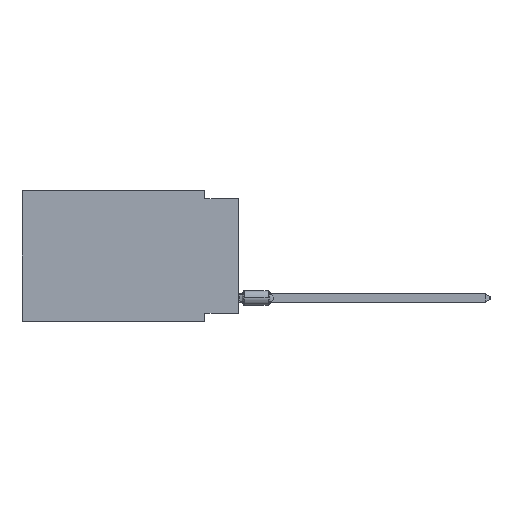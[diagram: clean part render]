
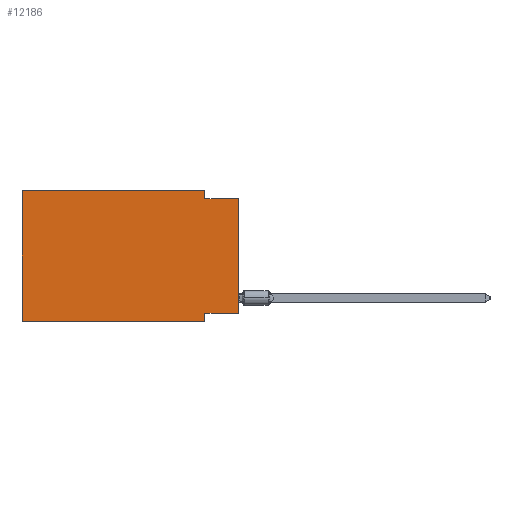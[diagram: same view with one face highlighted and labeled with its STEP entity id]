
A CAD part, left-side view. The second image highlights one B-rep face of the part: STEP entity #12186.
In plain terms, the highlighted planar face has unit normal (-1, 0, 0).
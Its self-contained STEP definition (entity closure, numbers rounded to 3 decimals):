
#16 = CARTESIAN_POINT ( 'NONE',  ( 0., 0., -0.635 ) ) ;
#1553 = DIRECTION ( 'NONE',  ( 0., 0., 1. ) ) ;
#1969 = EDGE_LOOP ( 'NONE', ( #14533, #6865, #28409, #47356, #5239, #27205, #57407, #11912 ) ) ;
#5239 = ORIENTED_EDGE ( 'NONE', *, *, #33198, .F. ) ;
#5409 = DIRECTION ( 'NONE',  ( 0., -1., 0. ) ) ;
#6129 = CARTESIAN_POINT ( 'NONE',  ( 0., 0., 0. ) ) ;
#6865 = ORIENTED_EDGE ( 'NONE', *, *, #43798, .F. ) ;
#7364 = VECTOR ( 'NONE', #43977, 1000. ) ;
#9691 = CARTESIAN_POINT ( 'NONE',  ( 0., 2.54, 0. ) ) ;
#11912 = ORIENTED_EDGE ( 'NONE', *, *, #61430, .F. ) ;
#12186 = ADVANCED_FACE ( 'NONE', ( #35207 ), #50902, .F. ) ;
#12616 = VECTOR ( 'NONE', #14151, 1000. ) ;
#13844 = DIRECTION ( 'NONE',  ( 0., 1., 0. ) ) ;
#14151 = DIRECTION ( 'NONE',  ( 0., -1., 0. ) ) ;
#14533 = ORIENTED_EDGE ( 'NONE', *, *, #33318, .T. ) ;
#15422 = CARTESIAN_POINT ( 'NONE',  ( 0., 16.383, -9.906 ) ) ;
#15964 = CARTESIAN_POINT ( 'NONE',  ( 0., 16.383, 0. ) ) ;
#16090 = DIRECTION ( 'NONE',  ( 0., 0., 1. ) ) ;
#17294 = EDGE_CURVE ( 'NONE', #62697, #54357, #19584, .T. ) ;
#18287 = VECTOR ( 'NONE', #25739, 1000. ) ;
#19584 = LINE ( 'NONE', #39155, #12616 ) ;
#19908 = VECTOR ( 'NONE', #16090, 1000. ) ;
#20481 = DIRECTION ( 'NONE',  ( 0., 0., -1. ) ) ;
#23140 = VERTEX_POINT ( 'NONE', #39452 ) ;
#23768 = VERTEX_POINT ( 'NONE', #35349 ) ;
#24410 = LINE ( 'NONE', #37907, #27496 ) ;
#25739 = DIRECTION ( 'NONE',  ( 0., 0., -1. ) ) ;
#27205 = ORIENTED_EDGE ( 'NONE', *, *, #17294, .T. ) ;
#27210 = EDGE_CURVE ( 'NONE', #23140, #43662, #30550, .T. ) ;
#27496 = VECTOR ( 'NONE', #13844, 1000. ) ;
#28409 = ORIENTED_EDGE ( 'NONE', *, *, #27210, .F. ) ;
#29242 = LINE ( 'NONE', #16, #7364 ) ;
#30550 = LINE ( 'NONE', #9691, #18287 ) ;
#31188 = VECTOR ( 'NONE', #1553, 1000. ) ;
#31927 = VECTOR ( 'NONE', #5409, 1000. ) ;
#33198 = EDGE_CURVE ( 'NONE', #62697, #51671, #35253, .T. ) ;
#33318 = EDGE_CURVE ( 'NONE', #23768, #45983, #59716, .T. ) ;
#35207 = FACE_OUTER_BOUND ( 'NONE', #1969, .T. ) ;
#35253 = LINE ( 'NONE', #54802, #31188 ) ;
#35349 = CARTESIAN_POINT ( 'NONE',  ( 0., 0., -9.271 ) ) ;
#35551 = LINE ( 'NONE', #49985, #40958 ) ;
#37907 = CARTESIAN_POINT ( 'NONE',  ( 0., 0., -9.271 ) ) ;
#39030 = CARTESIAN_POINT ( 'NONE',  ( 0., 2.54, -9.906 ) ) ;
#39155 = CARTESIAN_POINT ( 'NONE',  ( 0., 16.383, -9.906 ) ) ;
#39452 = CARTESIAN_POINT ( 'NONE',  ( 0., 2.54, 0. ) ) ;
#39737 = CARTESIAN_POINT ( 'NONE',  ( 0., 16.383, 0. ) ) ;
#40958 = VECTOR ( 'NONE', #20481, 1000. ) ;
#41948 = EDGE_CURVE ( 'NONE', #51671, #23140, #49040, .T. ) ;
#42097 = CARTESIAN_POINT ( 'NONE',  ( 0., 2.54, -0.635 ) ) ;
#43662 = VERTEX_POINT ( 'NONE', #42097 ) ;
#43798 = EDGE_CURVE ( 'NONE', #43662, #45983, #29242, .T. ) ;
#43977 = DIRECTION ( 'NONE',  ( 0., -1., 0. ) ) ;
#44375 = EDGE_CURVE ( 'NONE', #54690, #54357, #35551, .T. ) ;
#45983 = VERTEX_POINT ( 'NONE', #56425 ) ;
#47356 = ORIENTED_EDGE ( 'NONE', *, *, #41948, .F. ) ;
#48953 = CARTESIAN_POINT ( 'NONE',  ( 0., 2.54, -9.271 ) ) ;
#49040 = LINE ( 'NONE', #39737, #31927 ) ;
#49985 = CARTESIAN_POINT ( 'NONE',  ( 0., 2.54, -9.906 ) ) ;
#50902 = PLANE ( 'NONE',  #52243 ) ;
#51671 = VERTEX_POINT ( 'NONE', #53189 ) ;
#52243 = AXIS2_PLACEMENT_3D ( 'NONE', #15964, #60536, #60223 ) ;
#53189 = CARTESIAN_POINT ( 'NONE',  ( 0., 16.383, 0. ) ) ;
#54357 = VERTEX_POINT ( 'NONE', #39030 ) ;
#54690 = VERTEX_POINT ( 'NONE', #48953 ) ;
#54802 = CARTESIAN_POINT ( 'NONE',  ( 0., 16.383, 0. ) ) ;
#56425 = CARTESIAN_POINT ( 'NONE',  ( 0., 0., -0.635 ) ) ;
#57407 = ORIENTED_EDGE ( 'NONE', *, *, #44375, .F. ) ;
#59716 = LINE ( 'NONE', #6129, #19908 ) ;
#60223 = DIRECTION ( 'NONE',  ( 0., 0., -1. ) ) ;
#60536 = DIRECTION ( 'NONE',  ( 1., 0., 0. ) ) ;
#61430 = EDGE_CURVE ( 'NONE', #23768, #54690, #24410, .T. ) ;
#62697 = VERTEX_POINT ( 'NONE', #15422 ) ;
